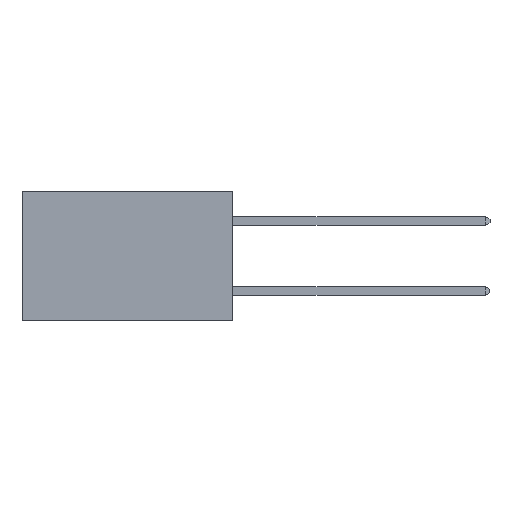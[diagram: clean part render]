
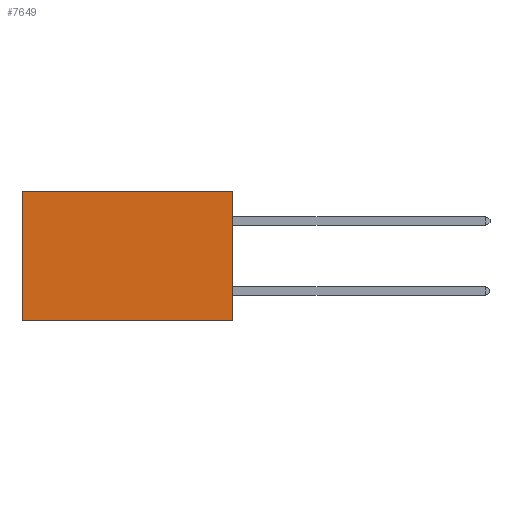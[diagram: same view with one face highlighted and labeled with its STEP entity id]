
A CAD part, left-side view. The second image highlights one B-rep face of the part: STEP entity #7649.
In plain terms, the highlighted planar face has unit normal (-1, 0, 0).
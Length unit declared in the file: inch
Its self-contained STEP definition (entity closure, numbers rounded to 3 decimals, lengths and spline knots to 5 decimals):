
#159 = CARTESIAN_POINT ( 'NONE',  ( 0.2875, 0.6, -0.37 ) ) ;
#1725 = CARTESIAN_POINT ( 'NONE',  ( 0.2875, 0., 0. ) ) ;
#3166 = DIRECTION ( 'NONE',  ( 0., 0., -1. ) ) ;
#3353 = ORIENTED_EDGE ( 'NONE', *, *, #16745, .T. ) ;
#3653 = CARTESIAN_POINT ( 'NONE',  ( 0.2875, 0.6, 0. ) ) ;
#4507 = ORIENTED_EDGE ( 'NONE', *, *, #10112, .F. ) ;
#4782 = VECTOR ( 'NONE', #9329, 39.37008 ) ;
#5021 = LINE ( 'NONE', #1725, #12134 ) ;
#5086 = DIRECTION ( 'NONE',  ( 0., 0., -1. ) ) ;
#5382 = CARTESIAN_POINT ( 'NONE',  ( 0.2875, 0., 0. ) ) ;
#6301 = ORIENTED_EDGE ( 'NONE', *, *, #12301, .T. ) ;
#6388 = FACE_OUTER_BOUND ( 'NONE', #17427, .T. ) ;
#6804 = DIRECTION ( 'NONE',  ( 0., 0., -1. ) ) ;
#6943 = VECTOR ( 'NONE', #8390, 39.37008 ) ;
#7392 = LINE ( 'NONE', #14048, #6943 ) ;
#7649 = ADVANCED_FACE ( 'NONE', ( #6388 ), #11064, .F. ) ;
#8178 = CARTESIAN_POINT ( 'NONE',  ( 0.2875, 0., -0.37 ) ) ;
#8390 = DIRECTION ( 'NONE',  ( 0., 1., 0. ) ) ;
#9329 = DIRECTION ( 'NONE',  ( 0., 1., 0. ) ) ;
#9392 = CARTESIAN_POINT ( 'NONE',  ( 0.2875, 0., -0.37 ) ) ;
#9765 = LINE ( 'NONE', #3653, #16405 ) ;
#9849 = EDGE_CURVE ( 'NONE', #17733, #10233, #5021, .T. ) ;
#10112 = EDGE_CURVE ( 'NONE', #10233, #12440, #15227, .T. ) ;
#10233 = VERTEX_POINT ( 'NONE', #8178 ) ;
#10240 = CARTESIAN_POINT ( 'NONE',  ( 0.2875, 0.6, 0. ) ) ;
#11064 = PLANE ( 'NONE',  #18122 ) ;
#12134 = VECTOR ( 'NONE', #3166, 39.37008 ) ;
#12301 = EDGE_CURVE ( 'NONE', #17733, #15246, #7392, .T. ) ;
#12440 = VERTEX_POINT ( 'NONE', #159 ) ;
#14048 = CARTESIAN_POINT ( 'NONE',  ( 0.2875, 0., 0. ) ) ;
#15227 = LINE ( 'NONE', #9392, #4782 ) ;
#15246 = VERTEX_POINT ( 'NONE', #10240 ) ;
#15311 = DIRECTION ( 'NONE',  ( 1., 0., 0. ) ) ;
#15844 = CARTESIAN_POINT ( 'NONE',  ( 0.2875, 0., 0. ) ) ;
#16405 = VECTOR ( 'NONE', #5086, 39.37008 ) ;
#16745 = EDGE_CURVE ( 'NONE', #15246, #12440, #9765, .T. ) ;
#17187 = ORIENTED_EDGE ( 'NONE', *, *, #9849, .F. ) ;
#17427 = EDGE_LOOP ( 'NONE', ( #3353, #4507, #17187, #6301 ) ) ;
#17733 = VERTEX_POINT ( 'NONE', #15844 ) ;
#18122 = AXIS2_PLACEMENT_3D ( 'NONE', #5382, #15311, #6804 ) ;
